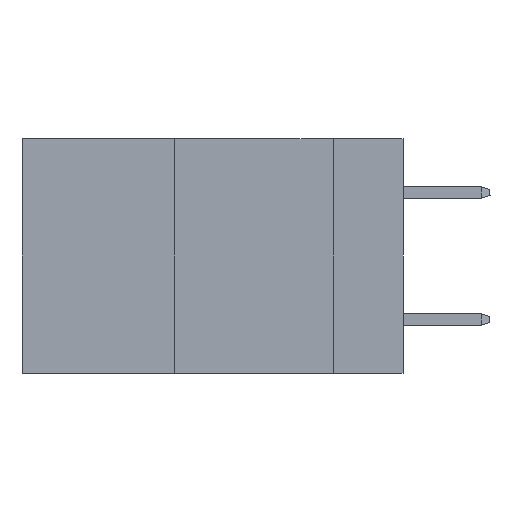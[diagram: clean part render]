
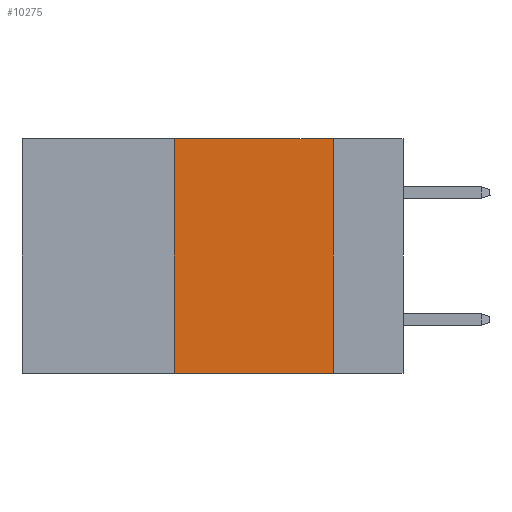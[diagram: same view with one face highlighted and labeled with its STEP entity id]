
A CAD part, left-side view. The second image highlights one B-rep face of the part: STEP entity #10275.
In plain terms, the highlighted planar face has unit normal (-1, 0, 0).
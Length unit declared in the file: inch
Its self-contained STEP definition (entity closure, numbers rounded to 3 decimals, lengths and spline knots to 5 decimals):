
#251 = VERTEX_POINT ( 'NONE', #25068 ) ;
#735 = CARTESIAN_POINT ( 'NONE',  ( 0., 0.36, 0. ) ) ;
#812 = CARTESIAN_POINT ( 'NONE',  ( 0., 0.6, 0. ) ) ;
#1630 = EDGE_LOOP ( 'NONE', ( #30217, #20950, #23203, #14436 ) ) ;
#4164 = VERTEX_POINT ( 'NONE', #12756 ) ;
#4683 = LINE ( 'NONE', #14485, #24117 ) ;
#4724 = EDGE_CURVE ( 'NONE', #25655, #251, #22849, .T. ) ;
#5835 = CARTESIAN_POINT ( 'NONE',  ( 0., 0.36, 0. ) ) ;
#6738 = AXIS2_PLACEMENT_3D ( 'NONE', #7879, #17670, #14484 ) ;
#7879 = CARTESIAN_POINT ( 'NONE',  ( 0., 0.6, 0. ) ) ;
#9892 = CARTESIAN_POINT ( 'NONE',  ( 0., 0.36, -0.37 ) ) ;
#10263 = FACE_OUTER_BOUND ( 'NONE', #1630, .T. ) ;
#10275 = ADVANCED_FACE ( 'NONE', ( #10263 ), #29873, .F. ) ;
#11236 = VERTEX_POINT ( 'NONE', #9892 ) ;
#12756 = CARTESIAN_POINT ( 'NONE',  ( 0., 0.11, -0.37 ) ) ;
#12952 = VECTOR ( 'NONE', #26694, 39.37008 ) ;
#14027 = CARTESIAN_POINT ( 'NONE',  ( 0., 0.6, -0.37 ) ) ;
#14436 = ORIENTED_EDGE ( 'NONE', *, *, #26809, .T. ) ;
#14484 = DIRECTION ( 'NONE',  ( 0., 0., -1. ) ) ;
#14485 = CARTESIAN_POINT ( 'NONE',  ( 0., 0.11, 0. ) ) ;
#17051 = DIRECTION ( 'NONE',  ( 0., 0., -1. ) ) ;
#17404 = LINE ( 'NONE', #5835, #27143 ) ;
#17670 = DIRECTION ( 'NONE',  ( 1., 0., 0. ) ) ;
#18997 = LINE ( 'NONE', #14027, #12952 ) ;
#20950 = ORIENTED_EDGE ( 'NONE', *, *, #4724, .F. ) ;
#22102 = VECTOR ( 'NONE', #27848, 39.37008 ) ;
#22580 = EDGE_CURVE ( 'NONE', #11236, #25655, #17404, .T. ) ;
#22849 = LINE ( 'NONE', #812, #22102 ) ;
#23203 = ORIENTED_EDGE ( 'NONE', *, *, #22580, .F. ) ;
#23735 = EDGE_CURVE ( 'NONE', #251, #4164, #4683, .T. ) ;
#24117 = VECTOR ( 'NONE', #17051, 39.37008 ) ;
#25068 = CARTESIAN_POINT ( 'NONE',  ( 0., 0.11, 0. ) ) ;
#25655 = VERTEX_POINT ( 'NONE', #735 ) ;
#26694 = DIRECTION ( 'NONE',  ( 0., -1., 0. ) ) ;
#26809 = EDGE_CURVE ( 'NONE', #11236, #4164, #18997, .T. ) ;
#27143 = VECTOR ( 'NONE', #27201, 39.37008 ) ;
#27201 = DIRECTION ( 'NONE',  ( 0., 0., 1. ) ) ;
#27848 = DIRECTION ( 'NONE',  ( 0., -1., 0. ) ) ;
#29873 = PLANE ( 'NONE',  #6738 ) ;
#30217 = ORIENTED_EDGE ( 'NONE', *, *, #23735, .F. ) ;
